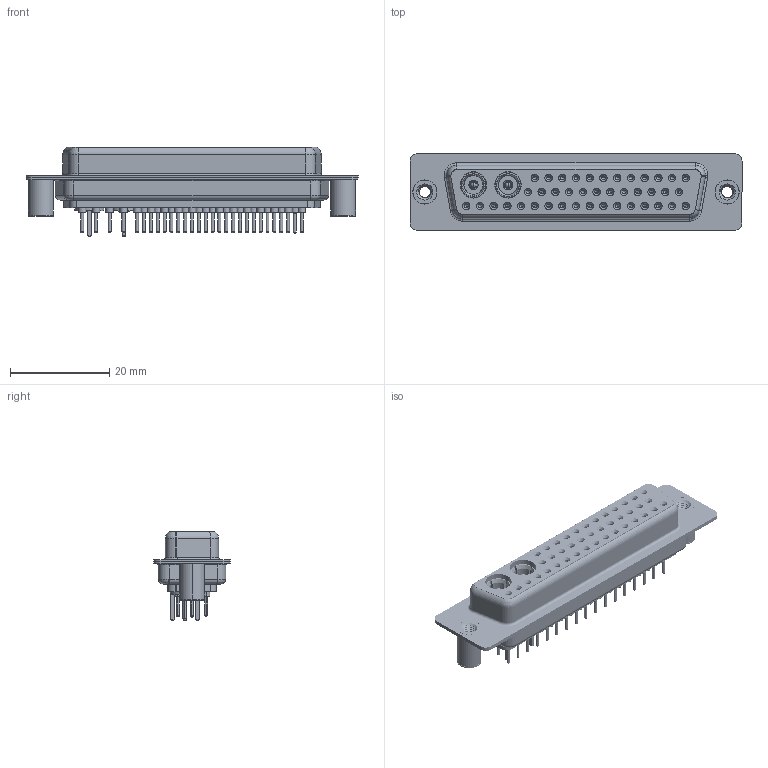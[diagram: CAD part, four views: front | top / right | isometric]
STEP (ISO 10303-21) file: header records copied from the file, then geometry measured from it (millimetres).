
FILE_DESCRIPTION (( 'STEP AP203' ), '1' );
FILE_NAME ('628-43W2624-5NB.STEP', '2019-06-26T21:22:48', ( '' ), ( '' ), 'SwSTEP 2.0', 'SolidWorks 2016', '' );
FILE_SCHEMA (( 'CONFIG_CONTROL_DESIGN' ));
Length unit declared in the file: millimetre
Products named in the file (13): 628Combo Threaded Board Spacer_B; 628Combo Shell Front_50 Contacts; Pin_Str; 628Combo Shell Rear_50 Contacts; Co-Ax Plug_Straight PC Tail; Insulator Pin_Straight PC Tail; 628Combo Contact Row 2_24; 628-43W2624-5NB; Locking Collar; 628Combo Contact Row 1_24; 628Combo Contact Row 3_24; 628Combo Housing_43W2; Co-Ax Plug Assy_St
Assembly tree (52 placements, depth 3):
  628-43W2624-5NB
    628Combo Housing_43W2
    628Combo Shell Front_50 Contacts
    628Combo Shell Rear_50 Contacts
    628Combo Threaded Board Spacer_B  x2
    628Combo Contact Row 1_24  x12
    628Combo Contact Row 2_24  x12
    628Combo Contact Row 3_24  x17
    Co-Ax Plug Assy_St  x2
      Co-Ax Plug_Straight PC Tail
      Insulator Pin_Straight PC Tail
      Pin_Str
      Locking Collar
Bounding box: 67 x 15.4 x 18.15 mm (x, y, z)
Volume: 7056.3 mm3; surface area: 15235.2 mm2
Topology: 54 solids, 54 shells, 2830 faces, 6567 edges, 4036 vertices
Faces by surface type: cylinder 1038, plane 796, torus 643, cone 335, bspline 10, sphere 8
Entity records: 35051 total; most frequent: CARTESIAN_POINT 7507, DIRECTION 5830, ORIENTED_EDGE 4808, AXIS2_PLACEMENT_3D 2461, EDGE_CURVE 2404, VERTEX_POINT 1524, CIRCLE 1352, EDGE_LOOP 1318
